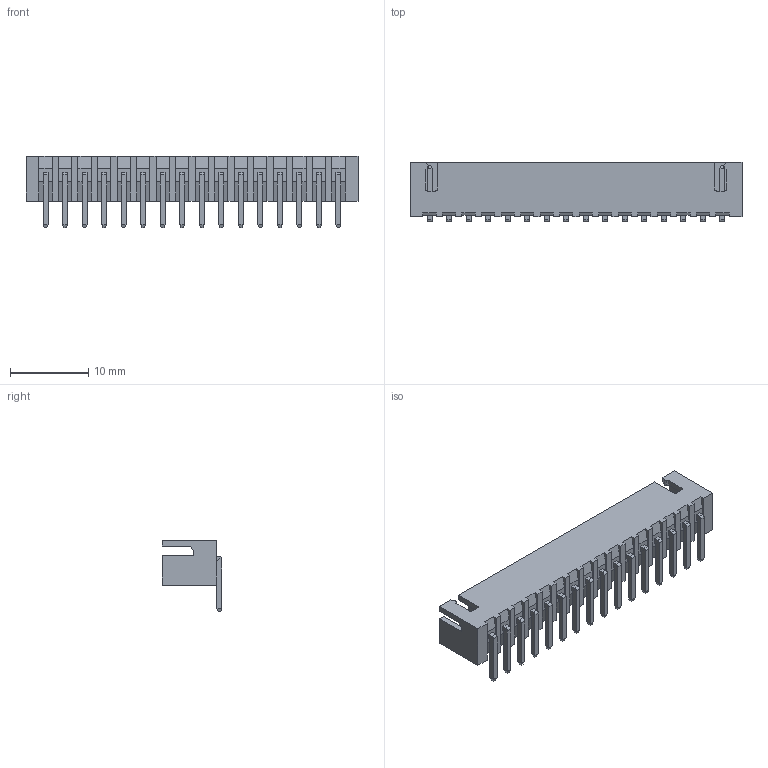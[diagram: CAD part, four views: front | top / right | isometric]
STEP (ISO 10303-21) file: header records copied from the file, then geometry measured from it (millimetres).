
FILE_DESCRIPTION (( 'STEP AP203' ), '1' );
FILE_NAME ('14K-516-416-AA1.STEP', '2024-02-23T17:48:08', ( '' ), ( '' ), 'SwSTEP 2.0', 'SolidWorks 2023', '' );
FILE_SCHEMA (( 'CONFIG_CONTROL_DESIGN' ));
Length unit declared in the file: millimetre
Products named in the file (3): 14K Series Pin_16; 14K-516-416-AA1; 14K Series Pin Header Insulator_516
Assembly tree (17 placements, depth 2):
  14K-516-416-AA1
    14K Series Pin Header Insulator_516
    14K Series Pin_16  x16
Bounding box: 42.5 x 7.64 x 9.15 mm (x, y, z)
Volume: 805.6 mm3; surface area: 2273.8 mm2
Topology: 17 solids, 17 shells, 552 faces, 1426 edges, 908 vertices
Faces by surface type: plane 511, cylinder 41
Entity records: 8041 total; most frequent: CARTESIAN_POINT 1316, ORIENTED_EDGE 1292, DIRECTION 1156, EDGE_CURVE 646, VECTOR 620, LINE 620, VERTEX_POINT 428, AXIS2_PLACEMENT_3D 268
